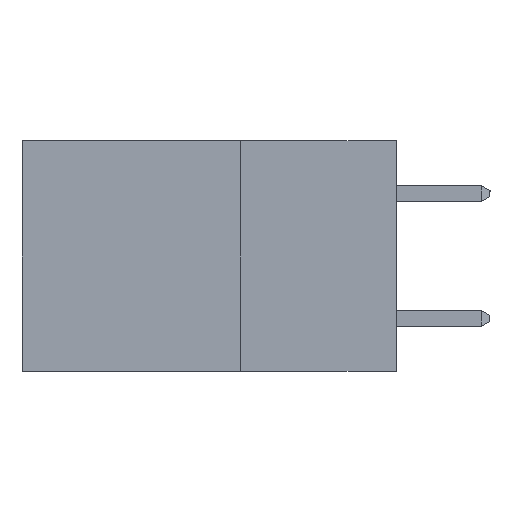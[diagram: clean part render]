
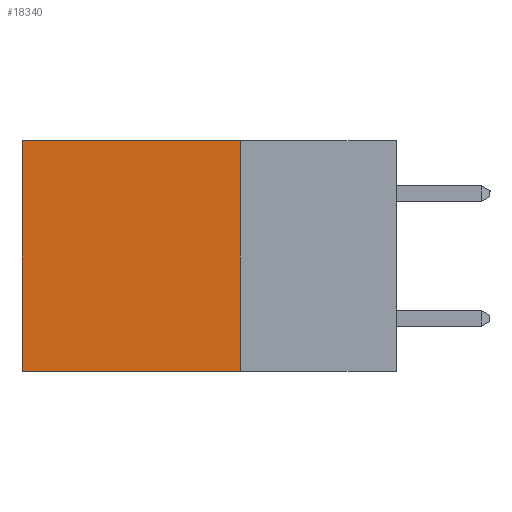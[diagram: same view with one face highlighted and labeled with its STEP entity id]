
A CAD part, left-side view. The second image highlights one B-rep face of the part: STEP entity #18340.
In plain terms, the highlighted planar face has unit normal (-1, 0, 0).
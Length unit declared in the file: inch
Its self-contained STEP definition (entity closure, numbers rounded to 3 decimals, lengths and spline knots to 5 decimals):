
#451 = CARTESIAN_POINT ( 'NONE',  ( 0.2615, 0.25, -0.37 ) ) ;
#2122 = CARTESIAN_POINT ( 'NONE',  ( 0.2615, 0.6, -0.37 ) ) ;
#2681 = EDGE_LOOP ( 'NONE', ( #9804, #10115, #11663, #17023 ) ) ;
#2687 = CARTESIAN_POINT ( 'NONE',  ( 0.2615, 0.25, -0.37 ) ) ;
#3144 = EDGE_CURVE ( 'NONE', #7963, #4387, #12115, .T. ) ;
#3153 = CARTESIAN_POINT ( 'NONE',  ( 0.2615, 0.25, -0.37 ) ) ;
#3560 = LINE ( 'NONE', #2122, #10385 ) ;
#3847 = DIRECTION ( 'NONE',  ( 0., 0., -1. ) ) ;
#3865 = EDGE_CURVE ( 'NONE', #4387, #4572, #17877, .T. ) ;
#3998 = CARTESIAN_POINT ( 'NONE',  ( 0.2615, 0.6, 0. ) ) ;
#4072 = CARTESIAN_POINT ( 'NONE',  ( 0.2615, 0.6, -0.37 ) ) ;
#4247 = VERTEX_POINT ( 'NONE', #3998 ) ;
#4387 = VERTEX_POINT ( 'NONE', #16049 ) ;
#4572 = VERTEX_POINT ( 'NONE', #4072 ) ;
#4798 = EDGE_CURVE ( 'NONE', #7963, #4247, #9230, .T. ) ;
#5212 = DIRECTION ( 'NONE',  ( 0., 1., 0. ) ) ;
#5229 = DIRECTION ( 'NONE',  ( 0., 0., -1. ) ) ;
#5976 = CARTESIAN_POINT ( 'NONE',  ( 0.2615, 0.25, 0. ) ) ;
#7963 = VERTEX_POINT ( 'NONE', #5976 ) ;
#9230 = LINE ( 'NONE', #13527, #14169 ) ;
#9804 = ORIENTED_EDGE ( 'NONE', *, *, #10730, .T. ) ;
#10115 = ORIENTED_EDGE ( 'NONE', *, *, #3865, .F. ) ;
#10385 = VECTOR ( 'NONE', #3847, 39.37008 ) ;
#10730 = EDGE_CURVE ( 'NONE', #4247, #4572, #3560, .T. ) ;
#11663 = ORIENTED_EDGE ( 'NONE', *, *, #3144, .F. ) ;
#12115 = LINE ( 'NONE', #451, #15940 ) ;
#12904 = DIRECTION ( 'NONE',  ( 1., 0., 0. ) ) ;
#13520 = AXIS2_PLACEMENT_3D ( 'NONE', #2687, #12904, #15701 ) ;
#13527 = CARTESIAN_POINT ( 'NONE',  ( 0.2615, 0.25, 0. ) ) ;
#14169 = VECTOR ( 'NONE', #5212, 39.37008 ) ;
#14352 = PLANE ( 'NONE',  #13520 ) ;
#14745 = VECTOR ( 'NONE', #17770, 39.37008 ) ;
#15701 = DIRECTION ( 'NONE',  ( 0., 0., -1. ) ) ;
#15940 = VECTOR ( 'NONE', #5229, 39.37008 ) ;
#16049 = CARTESIAN_POINT ( 'NONE',  ( 0.2615, 0.25, -0.37 ) ) ;
#17023 = ORIENTED_EDGE ( 'NONE', *, *, #4798, .T. ) ;
#17036 = FACE_OUTER_BOUND ( 'NONE', #2681, .T. ) ;
#17770 = DIRECTION ( 'NONE',  ( 0., 1., 0. ) ) ;
#17877 = LINE ( 'NONE', #3153, #14745 ) ;
#18340 = ADVANCED_FACE ( 'NONE', ( #17036 ), #14352, .F. ) ;
